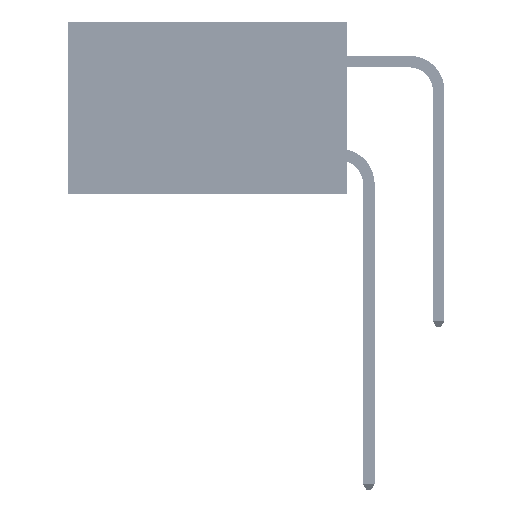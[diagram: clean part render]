
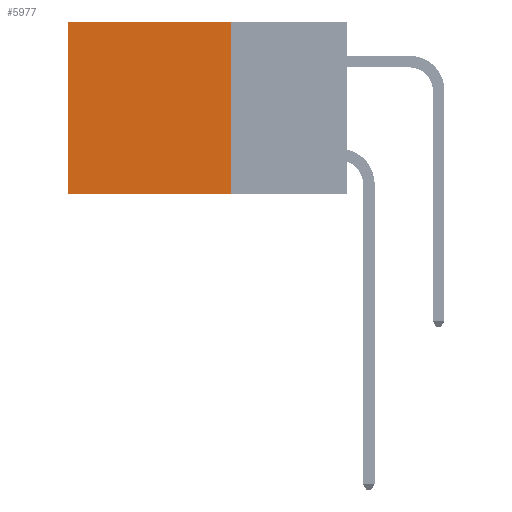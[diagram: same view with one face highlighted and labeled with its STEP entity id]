
A CAD part, left-side view. The second image highlights one B-rep face of the part: STEP entity #5977.
In plain terms, the highlighted planar face has unit normal (-1, 0, 0).
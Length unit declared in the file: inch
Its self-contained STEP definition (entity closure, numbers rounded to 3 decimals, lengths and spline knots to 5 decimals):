
#1110 = EDGE_CURVE ( 'NONE', #8575, #18971, #39573, .T. ) ;
#2540 = LINE ( 'NONE', #47168, #23782 ) ;
#2696 = CARTESIAN_POINT ( 'NONE',  ( 0.2875, 0.25, -0.37 ) ) ;
#5312 = AXIS2_PLACEMENT_3D ( 'NONE', #35844, #12093, #39805 ) ;
#5598 = VERTEX_POINT ( 'NONE', #37592 ) ;
#5667 = EDGE_CURVE ( 'NONE', #49981, #18971, #40551, .T. ) ;
#5977 = ADVANCED_FACE ( 'NONE', ( #24388 ), #8069, .F. ) ;
#8069 = PLANE ( 'NONE',  #5312 ) ;
#8574 = LINE ( 'NONE', #15222, #40227 ) ;
#8575 = VERTEX_POINT ( 'NONE', #2696 ) ;
#9834 = EDGE_CURVE ( 'NONE', #5598, #49981, #2540, .T. ) ;
#10160 = DIRECTION ( 'NONE',  ( 0., 0., -1. ) ) ;
#12093 = DIRECTION ( 'NONE',  ( 1., 0., 0. ) ) ;
#15222 = CARTESIAN_POINT ( 'NONE',  ( 0.2875, 0.25, 0. ) ) ;
#16711 = CARTESIAN_POINT ( 'NONE',  ( 0.2875, 0.6, 0. ) ) ;
#17905 = EDGE_CURVE ( 'NONE', #5598, #8575, #8574, .T. ) ;
#18971 = VERTEX_POINT ( 'NONE', #30766 ) ;
#19050 = DIRECTION ( 'NONE',  ( 0., 0., -1. ) ) ;
#23782 = VECTOR ( 'NONE', #51105, 39.37008 ) ;
#24388 = FACE_OUTER_BOUND ( 'NONE', #42794, .T. ) ;
#25480 = ORIENTED_EDGE ( 'NONE', *, *, #17905, .F. ) ;
#29373 = ORIENTED_EDGE ( 'NONE', *, *, #9834, .T. ) ;
#29996 = VECTOR ( 'NONE', #10160, 39.37008 ) ;
#30021 = CARTESIAN_POINT ( 'NONE',  ( 0.2875, 0.25, -0.37 ) ) ;
#30766 = CARTESIAN_POINT ( 'NONE',  ( 0.2875, 0.6, -0.37 ) ) ;
#35844 = CARTESIAN_POINT ( 'NONE',  ( 0.2875, 0.25, 0. ) ) ;
#37495 = ORIENTED_EDGE ( 'NONE', *, *, #5667, .T. ) ;
#37592 = CARTESIAN_POINT ( 'NONE',  ( 0.2875, 0.25, 0. ) ) ;
#37940 = CARTESIAN_POINT ( 'NONE',  ( 0.2875, 0.6, 0. ) ) ;
#39573 = LINE ( 'NONE', #30021, #40802 ) ;
#39805 = DIRECTION ( 'NONE',  ( 0., 0., -1. ) ) ;
#40227 = VECTOR ( 'NONE', #19050, 39.37008 ) ;
#40551 = LINE ( 'NONE', #37940, #29996 ) ;
#40802 = VECTOR ( 'NONE', #45562, 39.37008 ) ;
#42794 = EDGE_LOOP ( 'NONE', ( #37495, #50970, #25480, #29373 ) ) ;
#45562 = DIRECTION ( 'NONE',  ( 0., 1., 0. ) ) ;
#47168 = CARTESIAN_POINT ( 'NONE',  ( 0.2875, 0.25, 0. ) ) ;
#49981 = VERTEX_POINT ( 'NONE', #16711 ) ;
#50970 = ORIENTED_EDGE ( 'NONE', *, *, #1110, .F. ) ;
#51105 = DIRECTION ( 'NONE',  ( 0., 1., 0. ) ) ;
